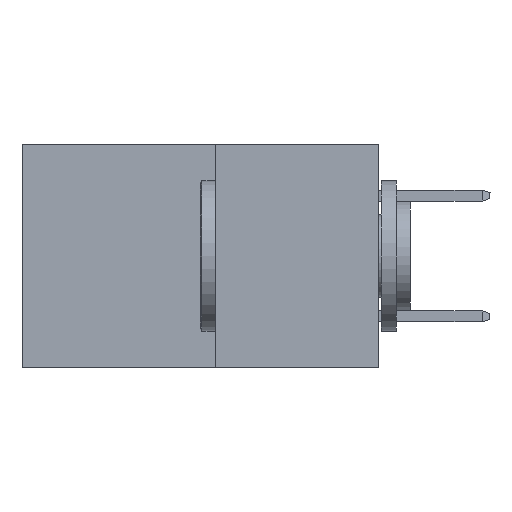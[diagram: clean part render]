
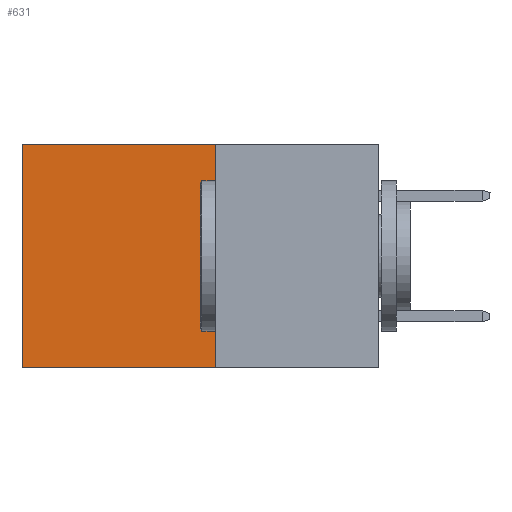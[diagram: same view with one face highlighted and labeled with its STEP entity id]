
A CAD part, left-side view. The second image highlights one B-rep face of the part: STEP entity #631.
In plain terms, the highlighted planar face has unit normal (-1, 0, 0).
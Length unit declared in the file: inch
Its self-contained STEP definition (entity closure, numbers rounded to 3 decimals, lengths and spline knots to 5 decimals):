
#145 = EDGE_CURVE ( 'NONE', #4597, #246, #6079, .T. ) ;
#169 = ORIENTED_EDGE ( 'NONE', *, *, #145, .T. ) ;
#246 = VERTEX_POINT ( 'NONE', #768 ) ;
#529 = FACE_OUTER_BOUND ( 'NONE', #4296, .T. ) ;
#603 = VERTEX_POINT ( 'NONE', #10266 ) ;
#631 = ADVANCED_FACE ( 'NONE', ( #529 ), #10098, .F. ) ;
#768 = CARTESIAN_POINT ( 'NONE',  ( 0.277, 0.59, 0. ) ) ;
#848 = DIRECTION ( 'NONE',  ( 0., 0., -1. ) ) ;
#964 = DIRECTION ( 'NONE',  ( 0., 0., -1. ) ) ;
#1015 = CARTESIAN_POINT ( 'NONE',  ( 0.277, 0.27, -0.37 ) ) ;
#1328 = CARTESIAN_POINT ( 'NONE',  ( 0.277, 0.59, -0.37 ) ) ;
#1404 = VERTEX_POINT ( 'NONE', #3037 ) ;
#1846 = DIRECTION ( 'NONE',  ( 0., 1., 0. ) ) ;
#1917 = VECTOR ( 'NONE', #3742, 39.37008 ) ;
#2046 = CARTESIAN_POINT ( 'NONE',  ( 0.277, 0.27, -0.37 ) ) ;
#3037 = CARTESIAN_POINT ( 'NONE',  ( 0.277, 0.27, -0.37 ) ) ;
#3464 = LINE ( 'NONE', #1015, #9513 ) ;
#3742 = DIRECTION ( 'NONE',  ( 0., 1., 0. ) ) ;
#4266 = EDGE_CURVE ( 'NONE', #246, #603, #8692, .T. ) ;
#4296 = EDGE_LOOP ( 'NONE', ( #5148, #6703, #5417, #169 ) ) ;
#4597 = VERTEX_POINT ( 'NONE', #9214 ) ;
#5148 = ORIENTED_EDGE ( 'NONE', *, *, #4266, .T. ) ;
#5235 = CARTESIAN_POINT ( 'NONE',  ( 0.277, 0.27, -0.37 ) ) ;
#5417 = ORIENTED_EDGE ( 'NONE', *, *, #5804, .F. ) ;
#5506 = VECTOR ( 'NONE', #1846, 39.37008 ) ;
#5804 = EDGE_CURVE ( 'NONE', #4597, #1404, #3464, .T. ) ;
#6074 = EDGE_CURVE ( 'NONE', #1404, #603, #9614, .T. ) ;
#6079 = LINE ( 'NONE', #8038, #1917 ) ;
#6588 = VECTOR ( 'NONE', #848, 39.37008 ) ;
#6703 = ORIENTED_EDGE ( 'NONE', *, *, #6074, .F. ) ;
#8038 = CARTESIAN_POINT ( 'NONE',  ( 0.277, 0.27, 0. ) ) ;
#8185 = DIRECTION ( 'NONE',  ( 0., 0., -1. ) ) ;
#8692 = LINE ( 'NONE', #1328, #6588 ) ;
#8964 = DIRECTION ( 'NONE',  ( 1., 0., 0. ) ) ;
#9034 = AXIS2_PLACEMENT_3D ( 'NONE', #2046, #8964, #8185 ) ;
#9214 = CARTESIAN_POINT ( 'NONE',  ( 0.277, 0.27, 0. ) ) ;
#9513 = VECTOR ( 'NONE', #964, 39.37008 ) ;
#9614 = LINE ( 'NONE', #5235, #5506 ) ;
#10098 = PLANE ( 'NONE',  #9034 ) ;
#10266 = CARTESIAN_POINT ( 'NONE',  ( 0.277, 0.59, -0.37 ) ) ;
